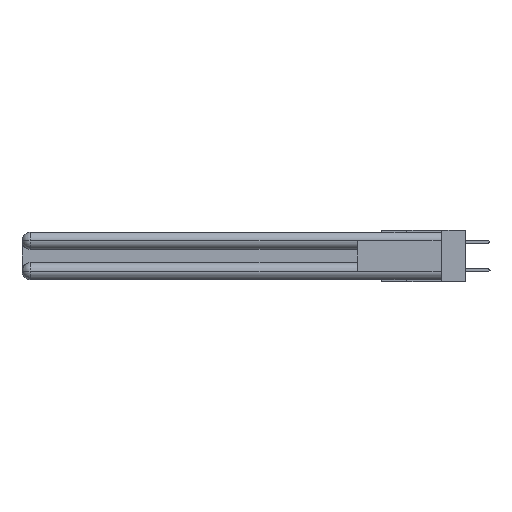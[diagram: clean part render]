
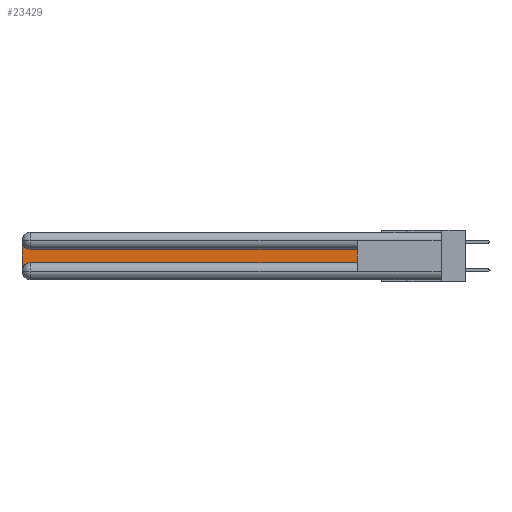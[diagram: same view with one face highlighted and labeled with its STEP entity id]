
A CAD part, left-side view. The second image highlights one B-rep face of the part: STEP entity #23429.
In plain terms, the highlighted planar face has unit normal (-1, 0, 0).
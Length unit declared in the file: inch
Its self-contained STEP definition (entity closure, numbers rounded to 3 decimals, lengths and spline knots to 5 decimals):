
#751 = VERTEX_POINT ( 'NONE', #22504 ) ;
#867 = CARTESIAN_POINT ( 'NONE',  ( 0.075, 0.6, -0.1225 ) ) ;
#1012 = LINE ( 'NONE', #867, #14468 ) ;
#1793 = EDGE_CURVE ( 'NONE', #21103, #5982, #20228, .T. ) ;
#2035 = AXIS2_PLACEMENT_3D ( 'NONE', #9682, #2898, #9787 ) ;
#2508 = VERTEX_POINT ( 'NONE', #24229 ) ;
#2898 = DIRECTION ( 'NONE',  ( 1., 0., 0. ) ) ;
#3704 = ORIENTED_EDGE ( 'NONE', *, *, #10369, .T. ) ;
#4319 = EDGE_CURVE ( 'NONE', #751, #21103, #1012, .T. ) ;
#4391 = EDGE_LOOP ( 'NONE', ( #16441, #29056, #7553, #25453, #19616, #3704 ) ) ;
#5099 = AXIS2_PLACEMENT_3D ( 'NONE', #28546, #21195, #9550 ) ;
#5982 = VERTEX_POINT ( 'NONE', #27474 ) ;
#6133 = CARTESIAN_POINT ( 'NONE',  ( 0.075, 2.94, -0.1225 ) ) ;
#6876 = DIRECTION ( 'NONE',  ( 1., 0., 0. ) ) ;
#7186 = VERTEX_POINT ( 'NONE', #26661 ) ;
#7553 = ORIENTED_EDGE ( 'NONE', *, *, #14118, .T. ) ;
#8578 = LINE ( 'NONE', #14022, #24244 ) ;
#9253 = VECTOR ( 'NONE', #25413, 39.37008 ) ;
#9550 = DIRECTION ( 'NONE',  ( 0., 0., -1. ) ) ;
#9587 = PLANE ( 'NONE',  #2035 ) ;
#9682 = CARTESIAN_POINT ( 'NONE',  ( 0.075, 3., -0.1225 ) ) ;
#9787 = DIRECTION ( 'NONE',  ( 0., 0., -1. ) ) ;
#10369 = EDGE_CURVE ( 'NONE', #2508, #751, #8578, .T. ) ;
#13409 = CARTESIAN_POINT ( 'NONE',  ( 0.075, 0.6, -0.2175 ) ) ;
#14022 = CARTESIAN_POINT ( 'NONE',  ( 0.075, 0.6, -0.2175 ) ) ;
#14118 = EDGE_CURVE ( 'NONE', #5982, #7186, #15821, .T. ) ;
#14468 = VECTOR ( 'NONE', #27075, 39.37008 ) ;
#15821 = LINE ( 'NONE', #17505, #30429 ) ;
#16139 = VERTEX_POINT ( 'NONE', #20335 ) ;
#16441 = ORIENTED_EDGE ( 'NONE', *, *, #4319, .T. ) ;
#17022 = EDGE_CURVE ( 'NONE', #7186, #16139, #20854, .T. ) ;
#17505 = CARTESIAN_POINT ( 'NONE',  ( 0.075, 3., -0.2175 ) ) ;
#18938 = CARTESIAN_POINT ( 'NONE',  ( 0.075, 2.94, -0.0625 ) ) ;
#19230 = EDGE_CURVE ( 'NONE', #16139, #2508, #27155, .T. ) ;
#19616 = ORIENTED_EDGE ( 'NONE', *, *, #19230, .T. ) ;
#20228 = CIRCLE ( 'NONE', #23383, 0.06 ) ;
#20335 = CARTESIAN_POINT ( 'NONE',  ( 0.075, 2.94, -0.2175 ) ) ;
#20854 = CIRCLE ( 'NONE', #5099, 0.06 ) ;
#21103 = VERTEX_POINT ( 'NONE', #6133 ) ;
#21195 = DIRECTION ( 'NONE',  ( 1., 0., 0. ) ) ;
#22504 = CARTESIAN_POINT ( 'NONE',  ( 0.075, 0.6, -0.1225 ) ) ;
#23134 = FACE_OUTER_BOUND ( 'NONE', #4391, .T. ) ;
#23383 = AXIS2_PLACEMENT_3D ( 'NONE', #18938, #6876, #23942 ) ;
#23429 = ADVANCED_FACE ( 'NONE', ( #23134 ), #9587, .F. ) ;
#23704 = DIRECTION ( 'NONE',  ( 0., 0., 1. ) ) ;
#23942 = DIRECTION ( 'NONE',  ( 0., 0., -1. ) ) ;
#24229 = CARTESIAN_POINT ( 'NONE',  ( 0.075, 0.6, -0.2175 ) ) ;
#24244 = VECTOR ( 'NONE', #23704, 39.37008 ) ;
#25413 = DIRECTION ( 'NONE',  ( 0., -1., 0. ) ) ;
#25453 = ORIENTED_EDGE ( 'NONE', *, *, #17022, .T. ) ;
#26661 = CARTESIAN_POINT ( 'NONE',  ( 0.075, 3., -0.2775 ) ) ;
#27075 = DIRECTION ( 'NONE',  ( 0., 1., 0. ) ) ;
#27155 = LINE ( 'NONE', #13409, #9253 ) ;
#27474 = CARTESIAN_POINT ( 'NONE',  ( 0.075, 3., -0.0625 ) ) ;
#28546 = CARTESIAN_POINT ( 'NONE',  ( 0.075, 2.94, -0.2775 ) ) ;
#29056 = ORIENTED_EDGE ( 'NONE', *, *, #1793, .T. ) ;
#29270 = DIRECTION ( 'NONE',  ( 0., 0., -1. ) ) ;
#30429 = VECTOR ( 'NONE', #29270, 39.37008 ) ;
